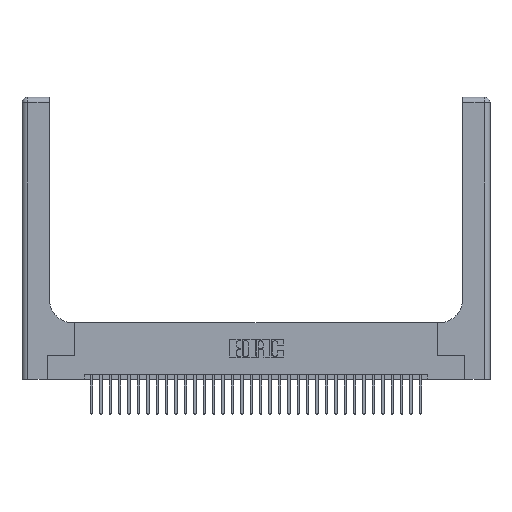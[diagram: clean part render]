
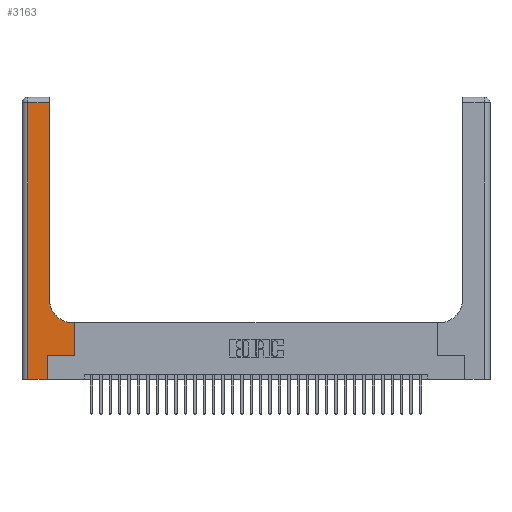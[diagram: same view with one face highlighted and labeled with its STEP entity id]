
A CAD part, top view. The second image highlights one B-rep face of the part: STEP entity #3163.
In plain terms, the highlighted planar face has unit normal (0, 0, 1).
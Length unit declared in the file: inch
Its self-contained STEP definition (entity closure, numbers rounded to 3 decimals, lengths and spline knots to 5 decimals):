
#689 = EDGE_CURVE ( 'NONE', #9187, #11495, #20171, .T. ) ;
#742 = CARTESIAN_POINT ( 'NONE',  ( 0.5585, 0.25, 0.37 ) ) ;
#957 = EDGE_CURVE ( 'NONE', #11495, #22610, #23826, .T. ) ;
#1068 = CARTESIAN_POINT ( 'NONE',  ( 0.2915, 0.85, 0.37 ) ) ;
#1586 = DIRECTION ( 'NONE',  ( 0., -1., 0. ) ) ;
#2334 = CARTESIAN_POINT ( 'NONE',  ( 0., 3., 0.37 ) ) ;
#2364 = VECTOR ( 'NONE', #24125, 39.37008 ) ;
#3163 = ADVANCED_FACE ( 'NONE', ( #9914 ), #25862, .F. ) ;
#3764 = CARTESIAN_POINT ( 'NONE',  ( 0.06, 0., 0.37 ) ) ;
#4002 = VERTEX_POINT ( 'NONE', #13270 ) ;
#4034 = EDGE_CURVE ( 'NONE', #4002, #13229, #29582, .T. ) ;
#4670 = VERTEX_POINT ( 'NONE', #24625 ) ;
#4720 = CIRCLE ( 'NONE', #12356, 0.25 ) ;
#5078 = VECTOR ( 'NONE', #13646, 39.37008 ) ;
#5143 = DIRECTION ( 'NONE',  ( 1., 0., 0. ) ) ;
#5255 = EDGE_CURVE ( 'NONE', #22610, #4002, #25052, .T. ) ;
#6193 = ORIENTED_EDGE ( 'NONE', *, *, #32596, .T. ) ;
#7581 = VECTOR ( 'NONE', #27396, 39.37008 ) ;
#7668 = DIRECTION ( 'NONE',  ( 0., 0., -1. ) ) ;
#7979 = VERTEX_POINT ( 'NONE', #15467 ) ;
#8472 = LINE ( 'NONE', #29558, #10595 ) ;
#8522 = CARTESIAN_POINT ( 'NONE',  ( 0.269, 0.25, 0.37 ) ) ;
#8660 = DIRECTION ( 'NONE',  ( 0., 1., 0. ) ) ;
#8967 = VECTOR ( 'NONE', #15713, 39.37008 ) ;
#9187 = VERTEX_POINT ( 'NONE', #23936 ) ;
#9914 = FACE_OUTER_BOUND ( 'NONE', #19096, .T. ) ;
#10394 = CARTESIAN_POINT ( 'NONE',  ( 0., 0., 0.37 ) ) ;
#10595 = VECTOR ( 'NONE', #8660, 39.37008 ) ;
#10674 = LINE ( 'NONE', #29611, #2364 ) ;
#11344 = VECTOR ( 'NONE', #25732, 39.37008 ) ;
#11495 = VERTEX_POINT ( 'NONE', #3764 ) ;
#12034 = EDGE_CURVE ( 'NONE', #22337, #32085, #8472, .T. ) ;
#12166 = LINE ( 'NONE', #742, #5078 ) ;
#12210 = CARTESIAN_POINT ( 'NONE',  ( 0.269, 0., 0.37 ) ) ;
#12356 = AXIS2_PLACEMENT_3D ( 'NONE', #21035, #26447, #5143 ) ;
#13053 = DIRECTION ( 'NONE',  ( 1., 0., 0. ) ) ;
#13229 = VERTEX_POINT ( 'NONE', #13744 ) ;
#13270 = CARTESIAN_POINT ( 'NONE',  ( 0.269, 0.25, 0.37 ) ) ;
#13379 = EDGE_CURVE ( 'NONE', #7979, #22337, #4720, .T. ) ;
#13646 = DIRECTION ( 'NONE',  ( 0., 1., 0. ) ) ;
#13744 = CARTESIAN_POINT ( 'NONE',  ( 0.5585, 0.25, 0.37 ) ) ;
#14885 = ORIENTED_EDGE ( 'NONE', *, *, #24028, .T. ) ;
#14915 = ORIENTED_EDGE ( 'NONE', *, *, #689, .T. ) ;
#15467 = CARTESIAN_POINT ( 'NONE',  ( 0.5415, 0.6, 0.37 ) ) ;
#15713 = DIRECTION ( 'NONE',  ( 1., 0., 0. ) ) ;
#17083 = EDGE_CURVE ( 'NONE', #32085, #9187, #26609, .T. ) ;
#18052 = CARTESIAN_POINT ( 'NONE',  ( 0.269, 0., 0.37 ) ) ;
#18242 = DIRECTION ( 'NONE',  ( -1., 0., 0. ) ) ;
#19096 = EDGE_LOOP ( 'NONE', ( #31704, #20870, #14915, #31683, #33657, #26971, #6193, #14885, #21866 ) ) ;
#19957 = CARTESIAN_POINT ( 'NONE',  ( 0.2915, 2.94, 0.37 ) ) ;
#20171 = LINE ( 'NONE', #20485, #29189 ) ;
#20485 = CARTESIAN_POINT ( 'NONE',  ( 0.06, 3., 0.37 ) ) ;
#20870 = ORIENTED_EDGE ( 'NONE', *, *, #17083, .T. ) ;
#21035 = CARTESIAN_POINT ( 'NONE',  ( 0.5415, 0.85, 0.37 ) ) ;
#21866 = ORIENTED_EDGE ( 'NONE', *, *, #13379, .T. ) ;
#22337 = VERTEX_POINT ( 'NONE', #1068 ) ;
#22610 = VERTEX_POINT ( 'NONE', #18052 ) ;
#23826 = LINE ( 'NONE', #10394, #26318 ) ;
#23936 = CARTESIAN_POINT ( 'NONE',  ( 0.06, 2.94, 0.37 ) ) ;
#24028 = EDGE_CURVE ( 'NONE', #4670, #7979, #10674, .T. ) ;
#24125 = DIRECTION ( 'NONE',  ( -1., 0., 0. ) ) ;
#24526 = AXIS2_PLACEMENT_3D ( 'NONE', #2334, #7668, #18242 ) ;
#24625 = CARTESIAN_POINT ( 'NONE',  ( 0.5585, 0.6, 0.37 ) ) ;
#24753 = CARTESIAN_POINT ( 'NONE',  ( 0., 2.94, 0.37 ) ) ;
#25052 = LINE ( 'NONE', #12210, #11344 ) ;
#25732 = DIRECTION ( 'NONE',  ( 0., 1., 0. ) ) ;
#25862 = PLANE ( 'NONE',  #24526 ) ;
#26318 = VECTOR ( 'NONE', #13053, 39.37008 ) ;
#26447 = DIRECTION ( 'NONE',  ( 0., 0., -1. ) ) ;
#26609 = LINE ( 'NONE', #24753, #7581 ) ;
#26971 = ORIENTED_EDGE ( 'NONE', *, *, #4034, .T. ) ;
#27396 = DIRECTION ( 'NONE',  ( -1., 0., 0. ) ) ;
#29189 = VECTOR ( 'NONE', #1586, 39.37008 ) ;
#29558 = CARTESIAN_POINT ( 'NONE',  ( 0.2915, 3., 0.37 ) ) ;
#29582 = LINE ( 'NONE', #8522, #8967 ) ;
#29611 = CARTESIAN_POINT ( 'NONE',  ( 0.2915, 0.6, 0.37 ) ) ;
#31683 = ORIENTED_EDGE ( 'NONE', *, *, #957, .T. ) ;
#31704 = ORIENTED_EDGE ( 'NONE', *, *, #12034, .T. ) ;
#32085 = VERTEX_POINT ( 'NONE', #19957 ) ;
#32596 = EDGE_CURVE ( 'NONE', #13229, #4670, #12166, .T. ) ;
#33657 = ORIENTED_EDGE ( 'NONE', *, *, #5255, .T. ) ;
